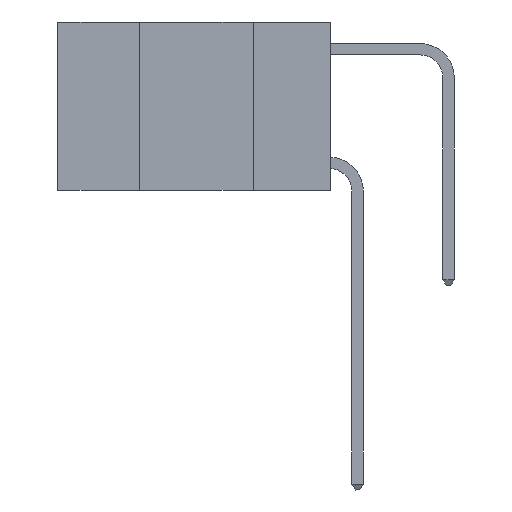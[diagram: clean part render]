
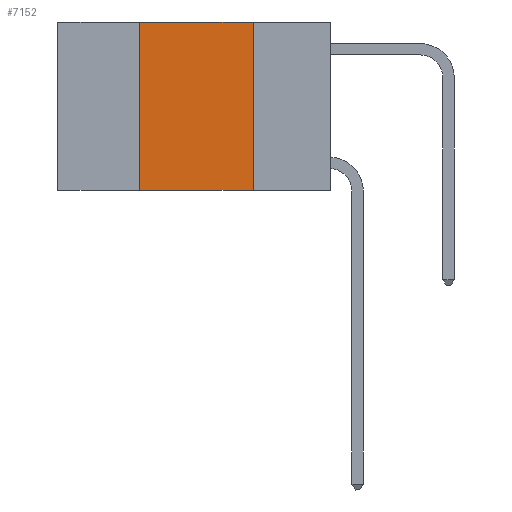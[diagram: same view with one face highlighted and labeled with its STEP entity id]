
A CAD part, left-side view. The second image highlights one B-rep face of the part: STEP entity #7152.
In plain terms, the highlighted planar face has unit normal (-1, 0, 0).
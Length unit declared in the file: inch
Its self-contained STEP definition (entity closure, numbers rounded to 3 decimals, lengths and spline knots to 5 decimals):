
#304 = CARTESIAN_POINT ( 'NONE',  ( 0., 0.6, 0. ) ) ;
#513 = VECTOR ( 'NONE', #6762, 39.37008 ) ;
#798 = VERTEX_POINT ( 'NONE', #4161 ) ;
#1048 = DIRECTION ( 'NONE',  ( 1., 0., 0. ) ) ;
#1753 = VERTEX_POINT ( 'NONE', #5790 ) ;
#3226 = PLANE ( 'NONE',  #10110 ) ;
#3996 = EDGE_LOOP ( 'NONE', ( #9152, #5234, #10345, #11065 ) ) ;
#4003 = VERTEX_POINT ( 'NONE', #10741 ) ;
#4127 = LINE ( 'NONE', #8271, #5741 ) ;
#4161 = CARTESIAN_POINT ( 'NONE',  ( 0., 0.42, 0. ) ) ;
#5062 = LINE ( 'NONE', #6908, #9875 ) ;
#5234 = ORIENTED_EDGE ( 'NONE', *, *, #11363, .F. ) ;
#5564 = EDGE_CURVE ( 'NONE', #4003, #798, #5062, .T. ) ;
#5741 = VECTOR ( 'NONE', #12422, 39.37008 ) ;
#5790 = CARTESIAN_POINT ( 'NONE',  ( 0., 0.17, 0. ) ) ;
#6301 = FACE_OUTER_BOUND ( 'NONE', #3996, .T. ) ;
#6762 = DIRECTION ( 'NONE',  ( 0., -1., 0. ) ) ;
#6908 = CARTESIAN_POINT ( 'NONE',  ( 0., 0.42, 0. ) ) ;
#7152 = ADVANCED_FACE ( 'NONE', ( #6301 ), #3226, .F. ) ;
#8131 = VERTEX_POINT ( 'NONE', #12960 ) ;
#8271 = CARTESIAN_POINT ( 'NONE',  ( 0., 0.17, 0. ) ) ;
#8727 = DIRECTION ( 'NONE',  ( 0., -1., 0. ) ) ;
#9152 = ORIENTED_EDGE ( 'NONE', *, *, #11233, .F. ) ;
#9438 = CARTESIAN_POINT ( 'NONE',  ( 0., 0.6, 0. ) ) ;
#9843 = LINE ( 'NONE', #304, #10951 ) ;
#9875 = VECTOR ( 'NONE', #10231, 39.37008 ) ;
#10110 = AXIS2_PLACEMENT_3D ( 'NONE', #9438, #1048, #10322 ) ;
#10231 = DIRECTION ( 'NONE',  ( 0., 0., 1. ) ) ;
#10322 = DIRECTION ( 'NONE',  ( 0., 0., -1. ) ) ;
#10345 = ORIENTED_EDGE ( 'NONE', *, *, #5564, .F. ) ;
#10741 = CARTESIAN_POINT ( 'NONE',  ( 0., 0.42, -0.37 ) ) ;
#10797 = CARTESIAN_POINT ( 'NONE',  ( 0., 0.6, -0.37 ) ) ;
#10951 = VECTOR ( 'NONE', #8727, 39.37008 ) ;
#11065 = ORIENTED_EDGE ( 'NONE', *, *, #11273, .T. ) ;
#11233 = EDGE_CURVE ( 'NONE', #1753, #8131, #4127, .T. ) ;
#11273 = EDGE_CURVE ( 'NONE', #4003, #8131, #11936, .T. ) ;
#11363 = EDGE_CURVE ( 'NONE', #798, #1753, #9843, .T. ) ;
#11936 = LINE ( 'NONE', #10797, #513 ) ;
#12422 = DIRECTION ( 'NONE',  ( 0., 0., -1. ) ) ;
#12960 = CARTESIAN_POINT ( 'NONE',  ( 0., 0.17, -0.37 ) ) ;
